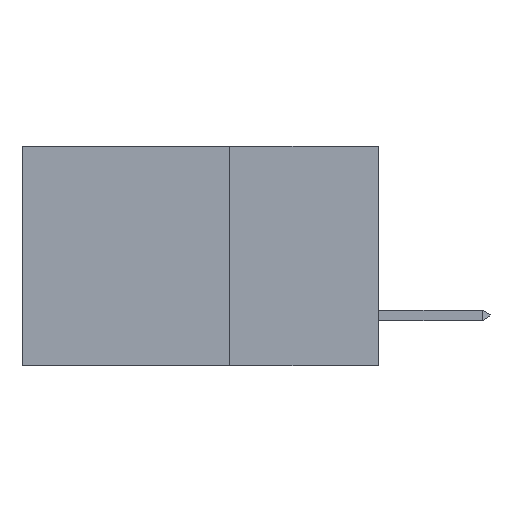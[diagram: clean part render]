
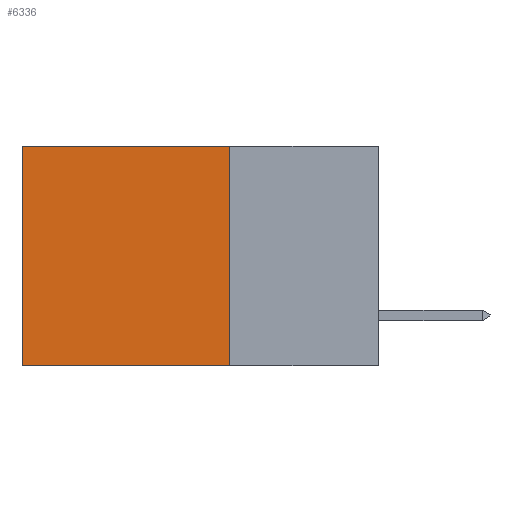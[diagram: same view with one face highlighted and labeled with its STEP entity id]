
A CAD part, left-side view. The second image highlights one B-rep face of the part: STEP entity #6336.
In plain terms, the highlighted planar face has unit normal (-1, 0, 0).
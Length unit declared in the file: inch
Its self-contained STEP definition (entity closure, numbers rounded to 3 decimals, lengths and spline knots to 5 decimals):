
#154 = CARTESIAN_POINT ( 'NONE',  ( 0.2615, 0.25, 0. ) ) ;
#432 = DIRECTION ( 'NONE',  ( 0., 0., -1. ) ) ;
#1029 = CARTESIAN_POINT ( 'NONE',  ( 0.2615, 0.6, 0. ) ) ;
#1057 = ORIENTED_EDGE ( 'NONE', *, *, #6200, .F. ) ;
#1387 = VERTEX_POINT ( 'NONE', #1029 ) ;
#1771 = LINE ( 'NONE', #154, #9163 ) ;
#2238 = VECTOR ( 'NONE', #432, 39.37008 ) ;
#2436 = LINE ( 'NONE', #8507, #4949 ) ;
#2617 = CARTESIAN_POINT ( 'NONE',  ( 0.2615, 0.6, -0.37 ) ) ;
#2662 = ORIENTED_EDGE ( 'NONE', *, *, #9407, .T. ) ;
#2766 = VECTOR ( 'NONE', #3413, 39.37008 ) ;
#3147 = EDGE_CURVE ( 'NONE', #1387, #10351, #3970, .T. ) ;
#3357 = VERTEX_POINT ( 'NONE', #4307 ) ;
#3413 = DIRECTION ( 'NONE',  ( 0., 0., -1. ) ) ;
#3717 = ORIENTED_EDGE ( 'NONE', *, *, #3147, .T. ) ;
#3970 = LINE ( 'NONE', #10149, #2238 ) ;
#4083 = DIRECTION ( 'NONE',  ( 0., 1., 0. ) ) ;
#4149 = CARTESIAN_POINT ( 'NONE',  ( 0.2615, 0.25, -0.37 ) ) ;
#4307 = CARTESIAN_POINT ( 'NONE',  ( 0.2615, 0.25, 0. ) ) ;
#4757 = ORIENTED_EDGE ( 'NONE', *, *, #5606, .F. ) ;
#4949 = VECTOR ( 'NONE', #4083, 39.37008 ) ;
#5228 = DIRECTION ( 'NONE',  ( 0., 1., 0. ) ) ;
#5606 = EDGE_CURVE ( 'NONE', #6856, #10351, #2436, .T. ) ;
#5715 = CARTESIAN_POINT ( 'NONE',  ( 0.2615, 0.25, -0.37 ) ) ;
#5908 = AXIS2_PLACEMENT_3D ( 'NONE', #4149, #8519, #10325 ) ;
#6200 = EDGE_CURVE ( 'NONE', #3357, #6856, #9579, .T. ) ;
#6336 = ADVANCED_FACE ( 'NONE', ( #11338 ), #6829, .F. ) ;
#6829 = PLANE ( 'NONE',  #5908 ) ;
#6856 = VERTEX_POINT ( 'NONE', #5715 ) ;
#8507 = CARTESIAN_POINT ( 'NONE',  ( 0.2615, 0.25, -0.37 ) ) ;
#8519 = DIRECTION ( 'NONE',  ( 1., 0., 0. ) ) ;
#9163 = VECTOR ( 'NONE', #5228, 39.37008 ) ;
#9407 = EDGE_CURVE ( 'NONE', #3357, #1387, #1771, .T. ) ;
#9448 = EDGE_LOOP ( 'NONE', ( #3717, #4757, #1057, #2662 ) ) ;
#9579 = LINE ( 'NONE', #10389, #2766 ) ;
#10149 = CARTESIAN_POINT ( 'NONE',  ( 0.2615, 0.6, -0.37 ) ) ;
#10325 = DIRECTION ( 'NONE',  ( 0., 0., -1. ) ) ;
#10351 = VERTEX_POINT ( 'NONE', #2617 ) ;
#10389 = CARTESIAN_POINT ( 'NONE',  ( 0.2615, 0.25, -0.37 ) ) ;
#11338 = FACE_OUTER_BOUND ( 'NONE', #9448, .T. ) ;
